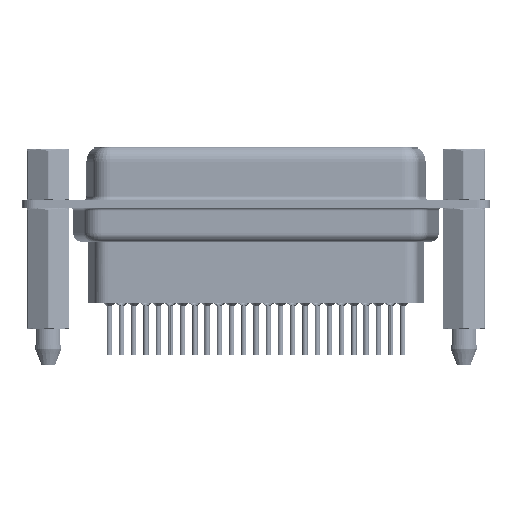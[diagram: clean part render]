
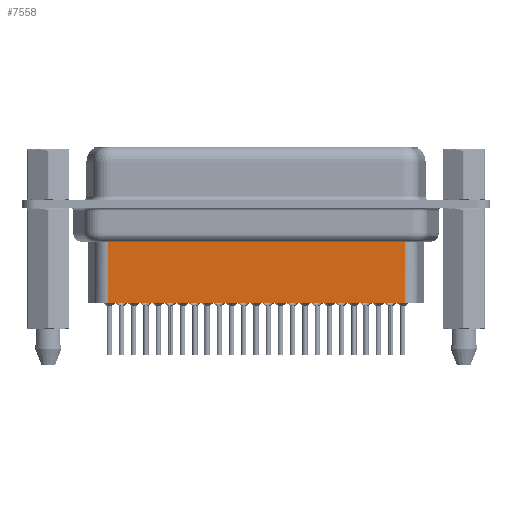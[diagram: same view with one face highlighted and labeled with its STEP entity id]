
A CAD part, front view. The second image highlights one B-rep face of the part: STEP entity #7558.
In plain terms, the highlighted planar face has unit normal (0, -1, 0).
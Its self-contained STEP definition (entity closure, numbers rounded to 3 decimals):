
#264 = CARTESIAN_POINT ( 'NONE',  ( 6.706, -3.5, -11.15 ) ) ;
#1552 = ORIENTED_EDGE ( 'NONE', *, *, #15422, .T. ) ;
#2290 = EDGE_LOOP ( 'NONE', ( #3460, #1552, #9044, #17207 ) ) ;
#2680 = CARTESIAN_POINT ( 'NONE',  ( 6.706, -3.5, -4.097 ) ) ;
#3460 = ORIENTED_EDGE ( 'NONE', *, *, #21295, .F. ) ;
#4389 = DIRECTION ( 'NONE',  ( 1., 0., 0. ) ) ;
#4510 = CARTESIAN_POINT ( 'NONE',  ( 40.344, -3.5, -4.097 ) ) ;
#5324 = VECTOR ( 'NONE', #8294, 1000. ) ;
#7516 = DIRECTION ( 'NONE',  ( 0., 0., -1. ) ) ;
#7558 = ADVANCED_FACE ( 'NONE', ( #12314 ), #9735, .T. ) ;
#7655 = VERTEX_POINT ( 'NONE', #2680 ) ;
#8294 = DIRECTION ( 'NONE',  ( 0., 0., -1. ) ) ;
#9044 = ORIENTED_EDGE ( 'NONE', *, *, #12485, .T. ) ;
#9269 = CARTESIAN_POINT ( 'NONE',  ( 6.459, -3.5, -4.097 ) ) ;
#9735 = PLANE ( 'NONE',  #21056 ) ;
#9925 = LINE ( 'NONE', #26190, #18189 ) ;
#9959 = VERTEX_POINT ( 'NONE', #264 ) ;
#12258 = VECTOR ( 'NONE', #25033, 1000. ) ;
#12314 = FACE_OUTER_BOUND ( 'NONE', #2290, .T. ) ;
#12485 = EDGE_CURVE ( 'NONE', #7655, #9959, #9925, .T. ) ;
#15098 = CARTESIAN_POINT ( 'NONE',  ( 40.344, -3.5, -11.15 ) ) ;
#15167 = EDGE_CURVE ( 'NONE', #23244, #9959, #29364, .T. ) ;
#15422 = EDGE_CURVE ( 'NONE', #20065, #7655, #32742, .T. ) ;
#17207 = ORIENTED_EDGE ( 'NONE', *, *, #15167, .F. ) ;
#18189 = VECTOR ( 'NONE', #7516, 1000. ) ;
#19058 = DIRECTION ( 'NONE',  ( -1., 0., 0. ) ) ;
#20065 = VERTEX_POINT ( 'NONE', #4510 ) ;
#21056 = AXIS2_PLACEMENT_3D ( 'NONE', #27548, #25153, #4389 ) ;
#21295 = EDGE_CURVE ( 'NONE', #20065, #23244, #33522, .T. ) ;
#22066 = VECTOR ( 'NONE', #19058, 1000. ) ;
#23244 = VERTEX_POINT ( 'NONE', #15098 ) ;
#23715 = CARTESIAN_POINT ( 'NONE',  ( 40.344, -3.5, -3.1 ) ) ;
#25033 = DIRECTION ( 'NONE',  ( -1., 0., 0. ) ) ;
#25153 = DIRECTION ( 'NONE',  ( 0., -1., 0. ) ) ;
#26190 = CARTESIAN_POINT ( 'NONE',  ( 6.706, -3.5, -3.1 ) ) ;
#27548 = CARTESIAN_POINT ( 'NONE',  ( 6.706, -3.5, -3.1 ) ) ;
#29364 = LINE ( 'NONE', #31922, #22066 ) ;
#31922 = CARTESIAN_POINT ( 'NONE',  ( 6.706, -3.5, -11.15 ) ) ;
#32742 = LINE ( 'NONE', #9269, #12258 ) ;
#33522 = LINE ( 'NONE', #23715, #5324 ) ;
